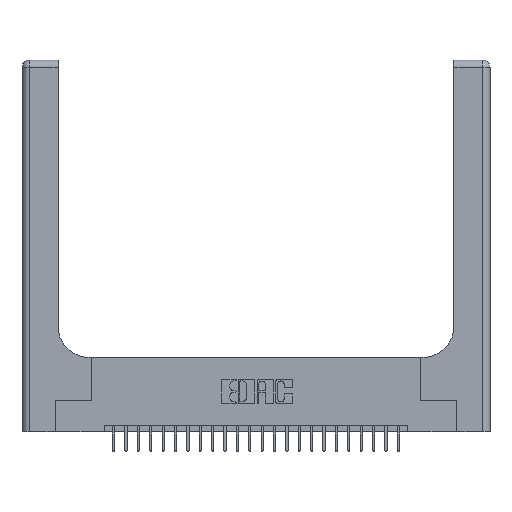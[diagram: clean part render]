
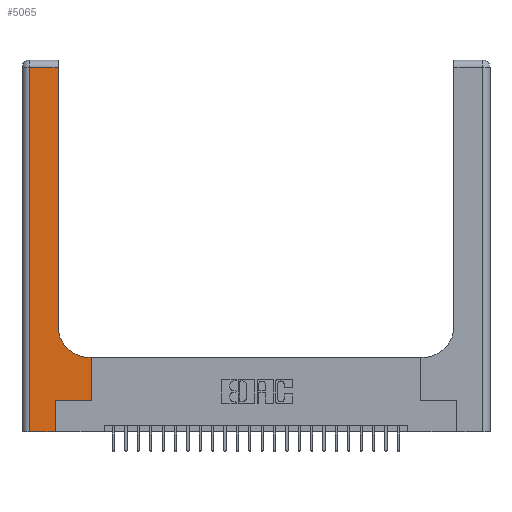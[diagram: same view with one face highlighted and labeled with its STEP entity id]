
A CAD part, top view. The second image highlights one B-rep face of the part: STEP entity #5065.
In plain terms, the highlighted planar face has unit normal (0, 0, 1).
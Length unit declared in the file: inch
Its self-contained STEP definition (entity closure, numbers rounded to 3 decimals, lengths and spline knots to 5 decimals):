
#83 = CARTESIAN_POINT ( 'NONE',  ( 0.5585, 0.6, 0.37 ) ) ;
#171 = CARTESIAN_POINT ( 'NONE',  ( 0.5415, 0.85, 0.37 ) ) ;
#481 = CARTESIAN_POINT ( 'NONE',  ( 0.06, 2.94, 0.37 ) ) ;
#676 = VERTEX_POINT ( 'NONE', #5755 ) ;
#980 = DIRECTION ( 'NONE',  ( 1., 0., 0. ) ) ;
#1004 = CARTESIAN_POINT ( 'NONE',  ( 0.2915, 0.85, 0.37 ) ) ;
#1132 = ORIENTED_EDGE ( 'NONE', *, *, #9473, .T. ) ;
#1506 = CARTESIAN_POINT ( 'NONE',  ( 0.269, 0.25, 0.37 ) ) ;
#1755 = ORIENTED_EDGE ( 'NONE', *, *, #21927, .T. ) ;
#2308 = DIRECTION ( 'NONE',  ( 1., 0., 0. ) ) ;
#2364 = VECTOR ( 'NONE', #12910, 39.37008 ) ;
#3916 = CARTESIAN_POINT ( 'NONE',  ( 0.2915, 3., 0.37 ) ) ;
#4314 = VECTOR ( 'NONE', #23473, 39.37008 ) ;
#4407 = DIRECTION ( 'NONE',  ( -1., 0., 0. ) ) ;
#5056 = EDGE_CURVE ( 'NONE', #12751, #12632, #5438, .T. ) ;
#5065 = ADVANCED_FACE ( 'NONE', ( #15611 ), #12549, .F. ) ;
#5267 = LINE ( 'NONE', #3916, #20213 ) ;
#5291 = CARTESIAN_POINT ( 'NONE',  ( 0.06, 0., 0.37 ) ) ;
#5438 = CIRCLE ( 'NONE', #13859, 0.25 ) ;
#5755 = CARTESIAN_POINT ( 'NONE',  ( 0.269, 0., 0.37 ) ) ;
#6018 = DIRECTION ( 'NONE',  ( 0., 1., 0. ) ) ;
#6080 = CARTESIAN_POINT ( 'NONE',  ( 0., 2.94, 0.37 ) ) ;
#6409 = VERTEX_POINT ( 'NONE', #481 ) ;
#6529 = VECTOR ( 'NONE', #980, 39.37008 ) ;
#7169 = CARTESIAN_POINT ( 'NONE',  ( 0.269, 0.25, 0.37 ) ) ;
#7327 = CARTESIAN_POINT ( 'NONE',  ( 0., 0., 0.37 ) ) ;
#7829 = LINE ( 'NONE', #6080, #23369 ) ;
#8257 = DIRECTION ( 'NONE',  ( -1., 0., 0. ) ) ;
#8968 = EDGE_CURVE ( 'NONE', #18299, #16290, #25993, .T. ) ;
#9473 = EDGE_CURVE ( 'NONE', #16290, #12751, #24069, .T. ) ;
#9905 = CARTESIAN_POINT ( 'NONE',  ( 0.5415, 0.6, 0.37 ) ) ;
#10018 = CARTESIAN_POINT ( 'NONE',  ( 0.06, 3., 0.37 ) ) ;
#10902 = EDGE_CURVE ( 'NONE', #13983, #18299, #17923, .T. ) ;
#11510 = EDGE_LOOP ( 'NONE', ( #26414, #20894, #1755, #24778, #16464, #23796, #23821, #1132, #20006 ) ) ;
#12549 = PLANE ( 'NONE',  #17888 ) ;
#12632 = VERTEX_POINT ( 'NONE', #1004 ) ;
#12684 = VERTEX_POINT ( 'NONE', #23605 ) ;
#12751 = VERTEX_POINT ( 'NONE', #9905 ) ;
#12910 = DIRECTION ( 'NONE',  ( -1., 0., 0. ) ) ;
#13677 = VECTOR ( 'NONE', #19453, 39.37008 ) ;
#13859 = AXIS2_PLACEMENT_3D ( 'NONE', #171, #14584, #2308 ) ;
#13983 = VERTEX_POINT ( 'NONE', #1506 ) ;
#14584 = DIRECTION ( 'NONE',  ( 0., 0., -1. ) ) ;
#14724 = VECTOR ( 'NONE', #24193, 39.37008 ) ;
#15066 = LINE ( 'NONE', #21439, #25260 ) ;
#15334 = LINE ( 'NONE', #10018, #14724 ) ;
#15611 = FACE_OUTER_BOUND ( 'NONE', #11510, .T. ) ;
#16290 = VERTEX_POINT ( 'NONE', #83 ) ;
#16464 = ORIENTED_EDGE ( 'NONE', *, *, #26338, .T. ) ;
#16574 = DIRECTION ( 'NONE',  ( 0., 0., -1. ) ) ;
#17152 = EDGE_CURVE ( 'NONE', #18879, #676, #19042, .T. ) ;
#17738 = CARTESIAN_POINT ( 'NONE',  ( 0.5585, 0.25, 0.37 ) ) ;
#17888 = AXIS2_PLACEMENT_3D ( 'NONE', #22651, #16574, #4407 ) ;
#17923 = LINE ( 'NONE', #7169, #6529 ) ;
#18299 = VERTEX_POINT ( 'NONE', #17738 ) ;
#18879 = VERTEX_POINT ( 'NONE', #5291 ) ;
#19042 = LINE ( 'NONE', #7327, #13677 ) ;
#19453 = DIRECTION ( 'NONE',  ( 1., 0., 0. ) ) ;
#19680 = EDGE_CURVE ( 'NONE', #12684, #6409, #7829, .T. ) ;
#20006 = ORIENTED_EDGE ( 'NONE', *, *, #5056, .T. ) ;
#20213 = VECTOR ( 'NONE', #6018, 39.37008 ) ;
#20894 = ORIENTED_EDGE ( 'NONE', *, *, #19680, .T. ) ;
#21439 = CARTESIAN_POINT ( 'NONE',  ( 0.269, 0., 0.37 ) ) ;
#21515 = CARTESIAN_POINT ( 'NONE',  ( 0.5585, 0.25, 0.37 ) ) ;
#21927 = EDGE_CURVE ( 'NONE', #6409, #18879, #15334, .T. ) ;
#22651 = CARTESIAN_POINT ( 'NONE',  ( 0., 3., 0.37 ) ) ;
#23017 = CARTESIAN_POINT ( 'NONE',  ( 0.2915, 0.6, 0.37 ) ) ;
#23369 = VECTOR ( 'NONE', #8257, 39.37008 ) ;
#23473 = DIRECTION ( 'NONE',  ( 0., 1., 0. ) ) ;
#23480 = DIRECTION ( 'NONE',  ( 0., 1., 0. ) ) ;
#23605 = CARTESIAN_POINT ( 'NONE',  ( 0.2915, 2.94, 0.37 ) ) ;
#23796 = ORIENTED_EDGE ( 'NONE', *, *, #10902, .T. ) ;
#23821 = ORIENTED_EDGE ( 'NONE', *, *, #8968, .T. ) ;
#24069 = LINE ( 'NONE', #23017, #2364 ) ;
#24130 = EDGE_CURVE ( 'NONE', #12632, #12684, #5267, .T. ) ;
#24193 = DIRECTION ( 'NONE',  ( 0., -1., 0. ) ) ;
#24778 = ORIENTED_EDGE ( 'NONE', *, *, #17152, .T. ) ;
#25260 = VECTOR ( 'NONE', #23480, 39.37008 ) ;
#25993 = LINE ( 'NONE', #21515, #4314 ) ;
#26338 = EDGE_CURVE ( 'NONE', #676, #13983, #15066, .T. ) ;
#26414 = ORIENTED_EDGE ( 'NONE', *, *, #24130, .T. ) ;
